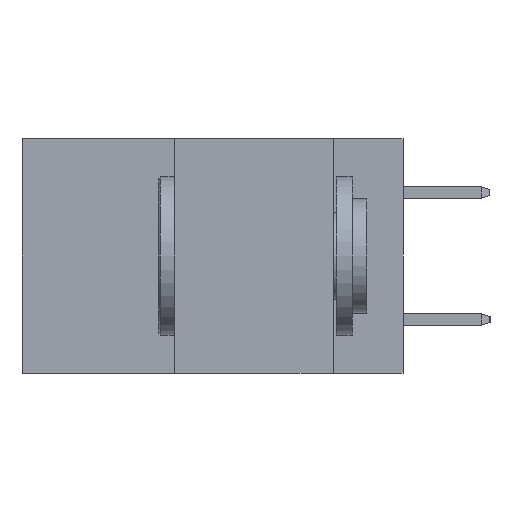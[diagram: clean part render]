
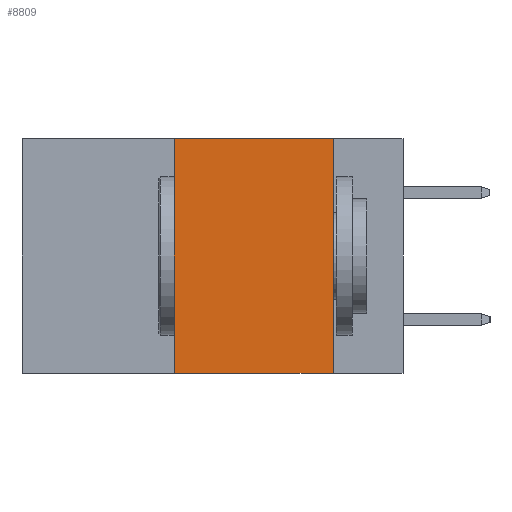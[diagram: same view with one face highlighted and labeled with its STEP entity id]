
A CAD part, left-side view. The second image highlights one B-rep face of the part: STEP entity #8809.
In plain terms, the highlighted planar face has unit normal (-1, 0, 0).
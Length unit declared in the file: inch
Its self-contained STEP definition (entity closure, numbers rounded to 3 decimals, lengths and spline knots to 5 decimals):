
#1205 = CARTESIAN_POINT ( 'NONE',  ( 0., 0.11, -0.37 ) ) ;
#1347 = DIRECTION ( 'NONE',  ( 0., 0., 1. ) ) ;
#1443 = FACE_OUTER_BOUND ( 'NONE', #9431, .T. ) ;
#1512 = VECTOR ( 'NONE', #8035, 39.37008 ) ;
#2813 = ORIENTED_EDGE ( 'NONE', *, *, #3291, .F. ) ;
#3140 = LINE ( 'NONE', #5464, #4472 ) ;
#3212 = ORIENTED_EDGE ( 'NONE', *, *, #7165, .T. ) ;
#3291 = EDGE_CURVE ( 'NONE', #9640, #4205, #4086, .T. ) ;
#3624 = VERTEX_POINT ( 'NONE', #6185 ) ;
#3720 = VECTOR ( 'NONE', #7857, 39.37008 ) ;
#3792 = LINE ( 'NONE', #4557, #7480 ) ;
#4086 = LINE ( 'NONE', #8559, #3720 ) ;
#4205 = VERTEX_POINT ( 'NONE', #7871 ) ;
#4357 = LINE ( 'NONE', #5053, #1512 ) ;
#4472 = VECTOR ( 'NONE', #4662, 39.37008 ) ;
#4557 = CARTESIAN_POINT ( 'NONE',  ( 0., 0.36, 0. ) ) ;
#4662 = DIRECTION ( 'NONE',  ( 0., -1., 0. ) ) ;
#5053 = CARTESIAN_POINT ( 'NONE',  ( 0., 0.11, 0. ) ) ;
#5261 = DIRECTION ( 'NONE',  ( 1., 0., 0. ) ) ;
#5464 = CARTESIAN_POINT ( 'NONE',  ( 0., 0.6, -0.37 ) ) ;
#5970 = ORIENTED_EDGE ( 'NONE', *, *, #7410, .F. ) ;
#6185 = CARTESIAN_POINT ( 'NONE',  ( 0., 0.36, -0.37 ) ) ;
#6773 = PLANE ( 'NONE',  #7334 ) ;
#7165 = EDGE_CURVE ( 'NONE', #3624, #8756, #3140, .T. ) ;
#7193 = ORIENTED_EDGE ( 'NONE', *, *, #8857, .F. ) ;
#7334 = AXIS2_PLACEMENT_3D ( 'NONE', #8288, #5261, #7371 ) ;
#7371 = DIRECTION ( 'NONE',  ( 0., 0., -1. ) ) ;
#7410 = EDGE_CURVE ( 'NONE', #4205, #8756, #4357, .T. ) ;
#7480 = VECTOR ( 'NONE', #1347, 39.37008 ) ;
#7857 = DIRECTION ( 'NONE',  ( 0., -1., 0. ) ) ;
#7871 = CARTESIAN_POINT ( 'NONE',  ( 0., 0.11, 0. ) ) ;
#8035 = DIRECTION ( 'NONE',  ( 0., 0., -1. ) ) ;
#8288 = CARTESIAN_POINT ( 'NONE',  ( 0., 0.6, 0. ) ) ;
#8559 = CARTESIAN_POINT ( 'NONE',  ( 0., 0.6, 0. ) ) ;
#8607 = CARTESIAN_POINT ( 'NONE',  ( 0., 0.36, 0. ) ) ;
#8756 = VERTEX_POINT ( 'NONE', #1205 ) ;
#8809 = ADVANCED_FACE ( 'NONE', ( #1443 ), #6773, .F. ) ;
#8857 = EDGE_CURVE ( 'NONE', #3624, #9640, #3792, .T. ) ;
#9431 = EDGE_LOOP ( 'NONE', ( #5970, #2813, #7193, #3212 ) ) ;
#9640 = VERTEX_POINT ( 'NONE', #8607 ) ;
